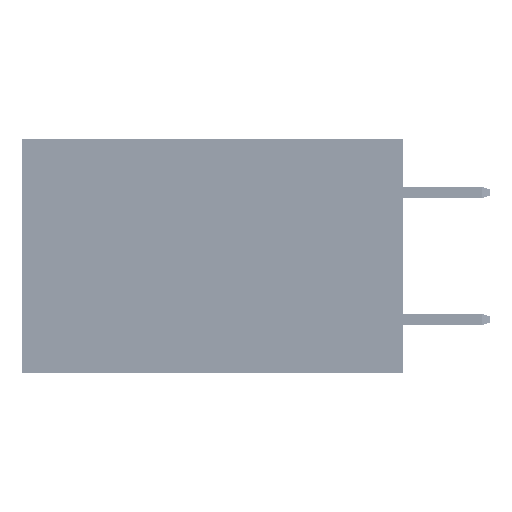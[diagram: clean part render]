
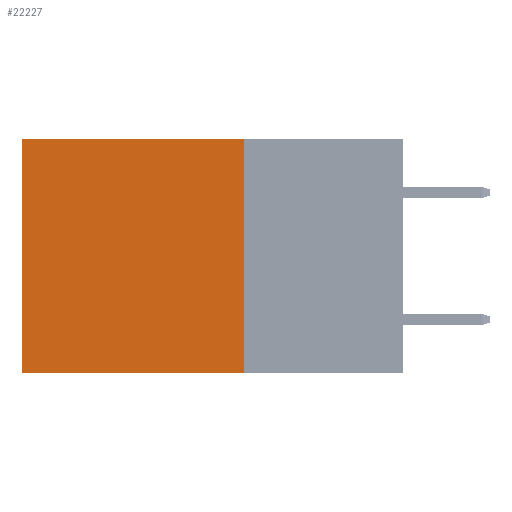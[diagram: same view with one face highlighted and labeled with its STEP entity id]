
A CAD part, left-side view. The second image highlights one B-rep face of the part: STEP entity #22227.
In plain terms, the highlighted planar face has unit normal (-1, 0, 0).
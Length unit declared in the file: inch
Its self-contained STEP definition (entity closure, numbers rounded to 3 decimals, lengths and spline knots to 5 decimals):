
#4947 = DIRECTION ( 'NONE',  ( 0., 0., -1. ) ) ;
#5747 = DIRECTION ( 'NONE',  ( 0., 1., 0. ) ) ;
#6746 = CARTESIAN_POINT ( 'NONE',  ( 0.2875, 0.25, -0.37 ) ) ;
#8635 = ORIENTED_EDGE ( 'NONE', *, *, #45238, .T. ) ;
#11131 = VECTOR ( 'NONE', #35871, 39.37008 ) ;
#11915 = DIRECTION ( 'NONE',  ( 0., 1., 0. ) ) ;
#12819 = CARTESIAN_POINT ( 'NONE',  ( 0.2875, 0.6, 0. ) ) ;
#13786 = ORIENTED_EDGE ( 'NONE', *, *, #14083, .F. ) ;
#14071 = DIRECTION ( 'NONE',  ( 1., 0., 0. ) ) ;
#14083 = EDGE_CURVE ( 'NONE', #46281, #34541, #33316, .T. ) ;
#14423 = CARTESIAN_POINT ( 'NONE',  ( 0.2875, 0.25, -0.37 ) ) ;
#17038 = EDGE_CURVE ( 'NONE', #37797, #46281, #34880, .T. ) ;
#22187 = CARTESIAN_POINT ( 'NONE',  ( 0.2875, 0.6, 0. ) ) ;
#22227 = ADVANCED_FACE ( 'NONE', ( #24449 ), #36030, .F. ) ;
#23155 = EDGE_LOOP ( 'NONE', ( #8635, #13786, #48083, #36230 ) ) ;
#24449 = FACE_OUTER_BOUND ( 'NONE', #23155, .T. ) ;
#27030 = EDGE_CURVE ( 'NONE', #37797, #37475, #32345, .T. ) ;
#28312 = VECTOR ( 'NONE', #4947, 39.37008 ) ;
#28707 = CARTESIAN_POINT ( 'NONE',  ( 0.2875, 0.25, 0. ) ) ;
#29043 = VECTOR ( 'NONE', #11915, 39.37008 ) ;
#29211 = DIRECTION ( 'NONE',  ( 0., 0., -1. ) ) ;
#32255 = CARTESIAN_POINT ( 'NONE',  ( 0.2875, 0.25, 0. ) ) ;
#32345 = LINE ( 'NONE', #46719, #29043 ) ;
#33316 = LINE ( 'NONE', #6746, #36079 ) ;
#34541 = VERTEX_POINT ( 'NONE', #35738 ) ;
#34880 = LINE ( 'NONE', #46478, #11131 ) ;
#35738 = CARTESIAN_POINT ( 'NONE',  ( 0.2875, 0.6, -0.37 ) ) ;
#35871 = DIRECTION ( 'NONE',  ( 0., 0., -1. ) ) ;
#36030 = PLANE ( 'NONE',  #43009 ) ;
#36079 = VECTOR ( 'NONE', #5747, 39.37008 ) ;
#36230 = ORIENTED_EDGE ( 'NONE', *, *, #27030, .T. ) ;
#37475 = VERTEX_POINT ( 'NONE', #22187 ) ;
#37797 = VERTEX_POINT ( 'NONE', #28707 ) ;
#40271 = LINE ( 'NONE', #12819, #28312 ) ;
#43009 = AXIS2_PLACEMENT_3D ( 'NONE', #32255, #14071, #29211 ) ;
#45238 = EDGE_CURVE ( 'NONE', #37475, #34541, #40271, .T. ) ;
#46281 = VERTEX_POINT ( 'NONE', #14423 ) ;
#46478 = CARTESIAN_POINT ( 'NONE',  ( 0.2875, 0.25, 0. ) ) ;
#46719 = CARTESIAN_POINT ( 'NONE',  ( 0.2875, 0.25, 0. ) ) ;
#48083 = ORIENTED_EDGE ( 'NONE', *, *, #17038, .F. ) ;
